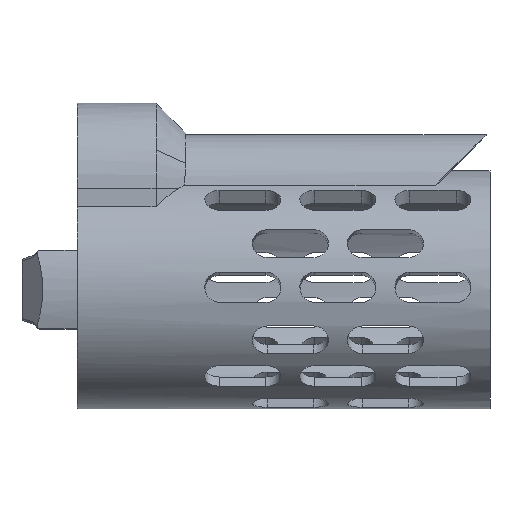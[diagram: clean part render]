
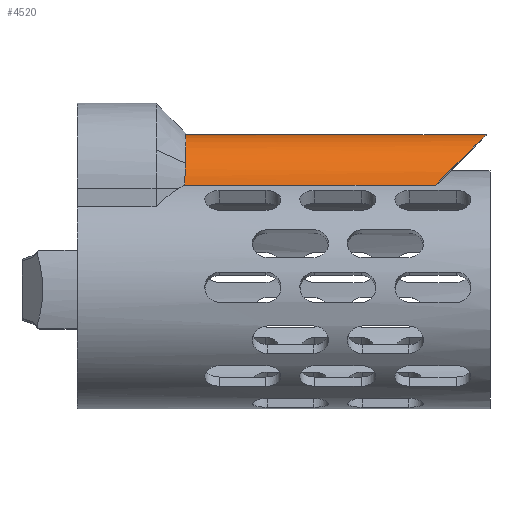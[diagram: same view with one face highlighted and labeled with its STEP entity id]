
A CAD part, top view. The second image highlights one B-rep face of the part: STEP entity #4520.
In plain terms, the highlighted cylindrical face has radius 13.5 mm (diameter 27 mm), a partial arc.
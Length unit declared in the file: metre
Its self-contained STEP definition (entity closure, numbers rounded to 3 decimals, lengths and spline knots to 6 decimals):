
#111=CIRCLE('',#4850,0.013539);
#112=CIRCLE('',#4851,0.013541);
#113=CIRCLE('',#4852,0.0135);
#267=B_SPLINE_CURVE_WITH_KNOTS('',3,(#7952,#7953,#7954,#7955),
 .UNSPECIFIED.,.F.,.F.,(4,4),(0.,1.),.UNSPECIFIED.);
#268=B_SPLINE_CURVE_WITH_KNOTS('',3,(#7959,#7960,#7961,#7962),
 .UNSPECIFIED.,.F.,.F.,(4,4),(4.792716,4.837685),
 .UNSPECIFIED.);
#269=B_SPLINE_CURVE_WITH_KNOTS('',3,(#7966,#7967,#7968,#7969),
 .UNSPECIFIED.,.F.,.F.,(4,4),(0.,1.),.UNSPECIFIED.);
#270=B_SPLINE_CURVE_WITH_KNOTS('',3,(#7973,#7974,#7975,#7976,#7977,#7978,
#7979,#7980,#7981,#7982,#7983,#7984,#7985,#7986,#7987,#7988,#7989,#7990,
#7991,#7992,#7993,#7994,#7995,#7996,#7997,#7998,#7999,#8000,#8001,#8002,
#8003,#8004,#8005,#8006,#8007,#8008),.UNSPECIFIED.,.F.,.F.,(4,1,1,1,1,1,
1,1,1,1,1,1,1,1,1,1,1,1,1,1,1,1,1,1,1,1,1,1,1,1,1,1,1,4),(0.,0.03125,0.0625,
0.09375,0.109375,0.117188,0.125,0.132813,0.140625,0.15625,0.1875,0.21875,
0.234375,0.25,0.265625,0.28125,0.3125,0.34375,0.375,0.40625,0.4375,0.5,
0.5625,0.625,0.6875,0.75,0.78125,0.8125,0.84375,0.875,0.890625,0.90625,
0.9375,1.),.UNSPECIFIED.);
#383=CYLINDRICAL_SURFACE('',#4849,0.0135);
#720=LINE('',#7957,#1096);
#721=LINE('',#7971,#1097);
#722=LINE('',#8010,#1098);
#1096=VECTOR('',#5776,1.);
#1097=VECTOR('',#5779,1.);
#1098=VECTOR('',#5780,1.);
#1930=ORIENTED_EDGE('',*,*,#2995,.F.);
#1931=ORIENTED_EDGE('',*,*,#2996,.T.);
#1932=ORIENTED_EDGE('',*,*,#2997,.T.);
#1933=ORIENTED_EDGE('',*,*,#2998,.F.);
#1934=ORIENTED_EDGE('',*,*,#2999,.T.);
#1935=ORIENTED_EDGE('',*,*,#3000,.F.);
#1936=ORIENTED_EDGE('',*,*,#3001,.T.);
#1937=ORIENTED_EDGE('',*,*,#3002,.F.);
#1938=ORIENTED_EDGE('',*,*,#3003,.F.);
#1939=ORIENTED_EDGE('',*,*,#3004,.F.);
#2995=EDGE_CURVE('',#3481,#3482,#111,.T.);
#2996=EDGE_CURVE('',#3481,#3483,#112,.T.);
#2997=EDGE_CURVE('',#3483,#3484,#267,.T.);
#2998=EDGE_CURVE('',#3485,#3484,#720,.T.);
#2999=EDGE_CURVE('',#3485,#3486,#268,.T.);
#3000=EDGE_CURVE('',#3487,#3486,#113,.T.);
#3001=EDGE_CURVE('',#3487,#3488,#269,.T.);
#3002=EDGE_CURVE('',#3489,#3488,#721,.T.);
#3003=EDGE_CURVE('',#3490,#3489,#270,.F.);
#3004=EDGE_CURVE('',#3482,#3490,#722,.T.);
#3481=VERTEX_POINT('',#7948);
#3482=VERTEX_POINT('',#7949);
#3483=VERTEX_POINT('',#7951);
#3484=VERTEX_POINT('',#7956);
#3485=VERTEX_POINT('',#7958);
#3486=VERTEX_POINT('',#7963);
#3487=VERTEX_POINT('',#7965);
#3488=VERTEX_POINT('',#7970);
#3489=VERTEX_POINT('',#7972);
#3490=VERTEX_POINT('',#8009);
#3782=EDGE_LOOP('',(#1930,#1931,#1932,#1933,#1934,#1935,#1936,#1937,#1938,
#1939));
#4108=FACE_BOUND('',#3782,.T.);
#4520=ADVANCED_FACE('',(#4108),#383,.T.);
#4849=AXIS2_PLACEMENT_3D('',#7946,#5770,#5771);
#4850=AXIS2_PLACEMENT_3D('',#7947,#5772,#5773);
#4851=AXIS2_PLACEMENT_3D('',#7950,#5774,#5775);
#4852=AXIS2_PLACEMENT_3D('',#7964,#5777,#5778);
#5770=DIRECTION('',(1.,0.,0.));
#5771=DIRECTION('',(0.,1.,0.));
#5772=DIRECTION('',(0.998,-0.062,-0.003));
#5773=DIRECTION('',(0.027,0.468,-0.884));
#5774=DIRECTION('',(-0.998,0.062,0.003));
#5775=DIRECTION('',(0.027,0.468,-0.884));
#5776=DIRECTION('',(1.,0.,0.));
#5777=DIRECTION('',(-1.,0.,0.));
#5778=DIRECTION('',(0.,1.,0.));
#5779=DIRECTION('',(-1.,0.,0.));
#5780=DIRECTION('',(1.,0.,0.));
#7946=CARTESIAN_POINT('',(0.037189,0.046521,0.001));
#7947=CARTESIAN_POINT('',(0.094912,0.046523,0.00104));
#7948=CARTESIAN_POINT('',(0.095273,0.052855,-0.010922));
#7949=CARTESIAN_POINT('',(0.095284,0.05303,-0.010827));
#7950=CARTESIAN_POINT('',(0.094913,0.046522,0.001041));
#7951=CARTESIAN_POINT('',(0.095261,0.052659,-0.011024));
#7952=CARTESIAN_POINT('',(0.095261,0.052659,-0.011024));
#7953=CARTESIAN_POINT('',(0.09518,0.052725,-0.010991));
#7954=CARTESIAN_POINT('',(0.095099,0.05279,-0.010957));
#7955=CARTESIAN_POINT('',(0.095018,0.052855,-0.010922));
#7956=CARTESIAN_POINT('',(0.095018,0.052855,-0.010922));
#7957=CARTESIAN_POINT('',(0.037189,0.052855,-0.010922));
#7958=CARTESIAN_POINT('',(0.037162,0.052855,-0.010922));
#7959=CARTESIAN_POINT('',(0.037162,0.052855,-0.010922));
#7960=CARTESIAN_POINT('',(0.037171,0.052995,-0.010848));
#7961=CARTESIAN_POINT('',(0.03718,0.053134,-0.01077));
#7962=CARTESIAN_POINT('',(0.037189,0.053272,-0.010691));
#7963=CARTESIAN_POINT('',(0.037189,0.053272,-0.010691));
#7964=CARTESIAN_POINT('',(0.037189,0.046521,0.001));
#7965=CARTESIAN_POINT('',(0.037189,0.053272,0.012691));
#7966=CARTESIAN_POINT('',(0.037189,0.053272,0.012691));
#7967=CARTESIAN_POINT('',(0.037114,0.052108,0.013363));
#7968=CARTESIAN_POINT('',(0.037006,0.050418,0.014123));
#7969=CARTESIAN_POINT('',(0.036865,0.048164,0.0144));
#7970=CARTESIAN_POINT('',(0.036865,0.048164,0.0144));
#7971=CARTESIAN_POINT('',(0.037189,0.048164,0.0144));
#7972=CARTESIAN_POINT('',(0.095831,0.048164,0.0144));
#7973=CARTESIAN_POINT('',(0.095831,0.048164,0.0144));
#7974=CARTESIAN_POINT('',(0.096253,0.048585,0.014348));
#7975=CARTESIAN_POINT('',(0.097055,0.049388,0.014209));
#7976=CARTESIAN_POINT('',(0.09814,0.05047,0.013924));
#7977=CARTESIAN_POINT('',(0.098947,0.051274,0.013643));
#7978=CARTESIAN_POINT('',(0.099454,0.051777,0.013436));
#7979=CARTESIAN_POINT('',(0.099739,0.052061,0.013311));
#7980=CARTESIAN_POINT('',(0.099916,0.052237,0.013231));
#7981=CARTESIAN_POINT('',(0.100198,0.052517,0.013096));
#7982=CARTESIAN_POINT('',(0.100529,0.052847,0.012929));
#7983=CARTESIAN_POINT('',(0.101107,0.053423,0.012613));
#7984=CARTESIAN_POINT('',(0.101876,0.054187,0.012129));
#7985=CARTESIAN_POINT('',(0.102577,0.054883,0.011608));
#7986=CARTESIAN_POINT('',(0.103104,0.055406,0.011168));
#7987=CARTESIAN_POINT('',(0.10346,0.055758,0.01085));
#7988=CARTESIAN_POINT('',(0.103872,0.056167,0.010451));
#7989=CARTESIAN_POINT('',(0.104369,0.05666,0.009926));
#7990=CARTESIAN_POINT('',(0.104949,0.057235,0.009238));
#7991=CARTESIAN_POINT('',(0.105565,0.057845,0.008374));
#7992=CARTESIAN_POINT('',(0.106091,0.058364,0.007509));
#7993=CARTESIAN_POINT('',(0.106586,0.058852,0.00653));
#7994=CARTESIAN_POINT('',(0.107118,0.059378,0.005218));
#7995=CARTESIAN_POINT('',(0.107582,0.059835,0.003543));
#7996=CARTESIAN_POINT('',(0.10782,0.060069,0.001424));
#7997=CARTESIAN_POINT('',(0.107721,0.059973,-0.000669));
#7998=CARTESIAN_POINT('',(0.107286,0.059543,-0.002761));
#7999=CARTESIAN_POINT('',(0.106672,0.058939,-0.004382));
#8000=CARTESIAN_POINT('',(0.105999,0.058273,-0.005672));
#8001=CARTESIAN_POINT('',(0.10545,0.05773,-0.006547));
#8002=CARTESIAN_POINT('',(0.104819,0.057106,-0.007401));
#8003=CARTESIAN_POINT('',(0.104235,0.056527,-0.008076));
#8004=CARTESIAN_POINT('',(0.103712,0.056008,-0.008609));
#8005=CARTESIAN_POINT('',(0.103221,0.055522,-0.009071));
#8006=CARTESIAN_POINT('',(0.102292,0.054601,-0.009855));
#8007=CARTESIAN_POINT('',(0.101377,0.05369,-0.010464));
#8008=CARTESIAN_POINT('',(0.100714,0.05303,-0.010827));
#8009=CARTESIAN_POINT('',(0.100714,0.05303,-0.010827));
#8010=CARTESIAN_POINT('',(0.0887,0.05303,-0.010827));
